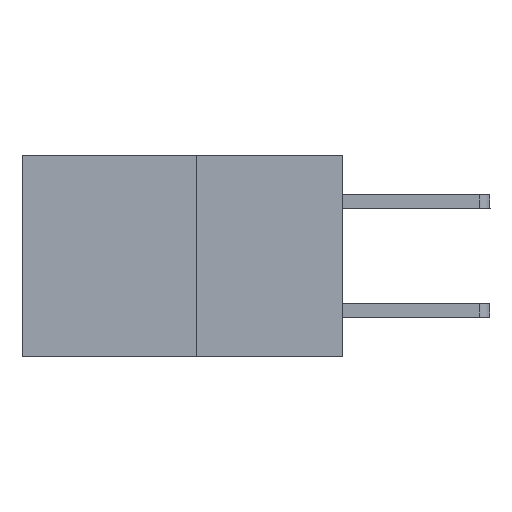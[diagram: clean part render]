
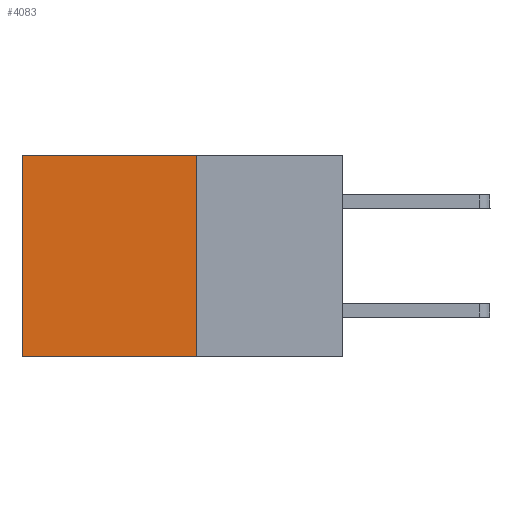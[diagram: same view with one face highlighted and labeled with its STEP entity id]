
A CAD part, left-side view. The second image highlights one B-rep face of the part: STEP entity #4083.
In plain terms, the highlighted planar face has unit normal (-1, 0, 0).
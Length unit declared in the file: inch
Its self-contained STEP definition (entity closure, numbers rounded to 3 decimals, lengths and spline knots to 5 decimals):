
#152 = CARTESIAN_POINT ( 'NONE',  ( 0.277, 0.27, -0.37 ) ) ;
#357 = DIRECTION ( 'NONE',  ( 0., 0., -1. ) ) ;
#392 = CARTESIAN_POINT ( 'NONE',  ( 0.277, 0.59, -0.37 ) ) ;
#617 = LINE ( 'NONE', #152, #8343 ) ;
#1259 = FACE_OUTER_BOUND ( 'NONE', #2371, .T. ) ;
#1271 = LINE ( 'NONE', #392, #9164 ) ;
#1405 = EDGE_CURVE ( 'NONE', #1768, #9842, #617, .T. ) ;
#1551 = CARTESIAN_POINT ( 'NONE',  ( 0.277, 0.27, 0. ) ) ;
#1768 = VERTEX_POINT ( 'NONE', #1551 ) ;
#1877 = VERTEX_POINT ( 'NONE', #8281 ) ;
#2061 = VECTOR ( 'NONE', #3581, 39.37008 ) ;
#2171 = DIRECTION ( 'NONE',  ( 0., 0., -1. ) ) ;
#2371 = EDGE_LOOP ( 'NONE', ( #6754, #8912, #5470, #9594 ) ) ;
#2898 = CARTESIAN_POINT ( 'NONE',  ( 0.277, 0.59, 0. ) ) ;
#2947 = LINE ( 'NONE', #7296, #4863 ) ;
#3581 = DIRECTION ( 'NONE',  ( 0., 1., 0. ) ) ;
#3623 = EDGE_CURVE ( 'NONE', #9165, #1877, #1271, .T. ) ;
#3649 = CARTESIAN_POINT ( 'NONE',  ( 0.277, 0.27, 0. ) ) ;
#4083 = ADVANCED_FACE ( 'NONE', ( #1259 ), #9183, .F. ) ;
#4298 = EDGE_CURVE ( 'NONE', #9842, #1877, #2947, .T. ) ;
#4863 = VECTOR ( 'NONE', #7252, 39.37008 ) ;
#5470 = ORIENTED_EDGE ( 'NONE', *, *, #1405, .F. ) ;
#5881 = AXIS2_PLACEMENT_3D ( 'NONE', #9541, #8855, #8755 ) ;
#6088 = EDGE_CURVE ( 'NONE', #1768, #9165, #8224, .T. ) ;
#6754 = ORIENTED_EDGE ( 'NONE', *, *, #3623, .T. ) ;
#7252 = DIRECTION ( 'NONE',  ( 0., 1., 0. ) ) ;
#7296 = CARTESIAN_POINT ( 'NONE',  ( 0.277, 0.27, -0.37 ) ) ;
#8193 = CARTESIAN_POINT ( 'NONE',  ( 0.277, 0.27, -0.37 ) ) ;
#8224 = LINE ( 'NONE', #3649, #2061 ) ;
#8281 = CARTESIAN_POINT ( 'NONE',  ( 0.277, 0.59, -0.37 ) ) ;
#8343 = VECTOR ( 'NONE', #2171, 39.37008 ) ;
#8755 = DIRECTION ( 'NONE',  ( 0., 0., -1. ) ) ;
#8855 = DIRECTION ( 'NONE',  ( 1., 0., 0. ) ) ;
#8912 = ORIENTED_EDGE ( 'NONE', *, *, #4298, .F. ) ;
#9164 = VECTOR ( 'NONE', #357, 39.37008 ) ;
#9165 = VERTEX_POINT ( 'NONE', #2898 ) ;
#9183 = PLANE ( 'NONE',  #5881 ) ;
#9541 = CARTESIAN_POINT ( 'NONE',  ( 0.277, 0.27, -0.37 ) ) ;
#9594 = ORIENTED_EDGE ( 'NONE', *, *, #6088, .T. ) ;
#9842 = VERTEX_POINT ( 'NONE', #8193 ) ;
